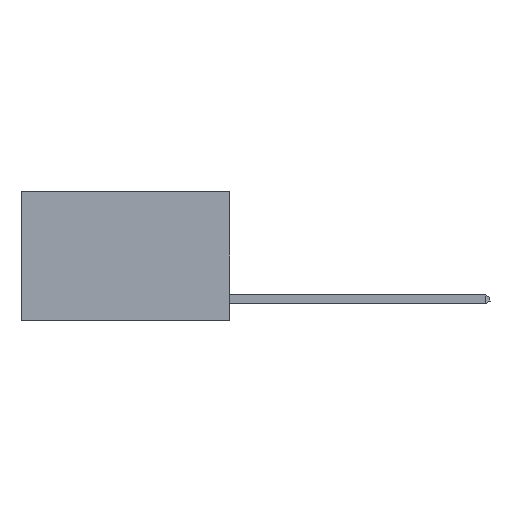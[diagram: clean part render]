
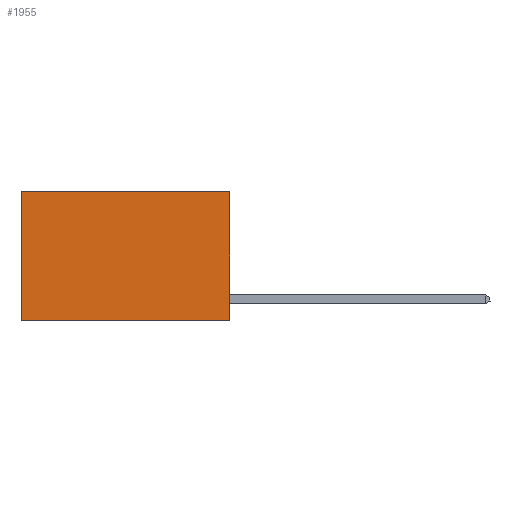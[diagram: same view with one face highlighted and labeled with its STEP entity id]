
A CAD part, left-side view. The second image highlights one B-rep face of the part: STEP entity #1955.
In plain terms, the highlighted planar face has unit normal (-1, 0, 0).
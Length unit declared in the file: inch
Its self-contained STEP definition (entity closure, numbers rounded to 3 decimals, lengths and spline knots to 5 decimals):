
#59 = LINE ( 'NONE', #3723, #6686 ) ;
#368 = DIRECTION ( 'NONE',  ( 0., 0., -1. ) ) ;
#416 = CARTESIAN_POINT ( 'NONE',  ( 0.2625, 0.6, 0. ) ) ;
#532 = VERTEX_POINT ( 'NONE', #5235 ) ;
#1898 = FACE_OUTER_BOUND ( 'NONE', #8113, .T. ) ;
#1925 = VECTOR ( 'NONE', #6934, 39.37008 ) ;
#1955 = ADVANCED_FACE ( 'NONE', ( #1898 ), #10443, .F. ) ;
#1997 = VECTOR ( 'NONE', #5068, 39.37008 ) ;
#2147 = CARTESIAN_POINT ( 'NONE',  ( 0.2625, 0., 0. ) ) ;
#2485 = AXIS2_PLACEMENT_3D ( 'NONE', #2147, #2920, #368 ) ;
#2717 = LINE ( 'NONE', #2907, #1925 ) ;
#2907 = CARTESIAN_POINT ( 'NONE',  ( 0.2625, 0., -0.37 ) ) ;
#2920 = DIRECTION ( 'NONE',  ( 1., 0., 0. ) ) ;
#3299 = ORIENTED_EDGE ( 'NONE', *, *, #6671, .F. ) ;
#3723 = CARTESIAN_POINT ( 'NONE',  ( 0.2625, 0.6, 0. ) ) ;
#4108 = ORIENTED_EDGE ( 'NONE', *, *, #7429, .T. ) ;
#4578 = VERTEX_POINT ( 'NONE', #9314 ) ;
#4613 = LINE ( 'NONE', #8494, #6379 ) ;
#5068 = DIRECTION ( 'NONE',  ( 0., 0., -1. ) ) ;
#5235 = CARTESIAN_POINT ( 'NONE',  ( 0.2625, 0.6, -0.37 ) ) ;
#6025 = DIRECTION ( 'NONE',  ( 0., 1., 0. ) ) ;
#6379 = VECTOR ( 'NONE', #6025, 39.37008 ) ;
#6627 = ORIENTED_EDGE ( 'NONE', *, *, #7870, .T. ) ;
#6668 = LINE ( 'NONE', #7596, #1997 ) ;
#6671 = EDGE_CURVE ( 'NONE', #8196, #532, #2717, .T. ) ;
#6686 = VECTOR ( 'NONE', #7843, 39.37008 ) ;
#6934 = DIRECTION ( 'NONE',  ( 0., 1., 0. ) ) ;
#7429 = EDGE_CURVE ( 'NONE', #9465, #532, #59, .T. ) ;
#7596 = CARTESIAN_POINT ( 'NONE',  ( 0.2625, 0., 0. ) ) ;
#7843 = DIRECTION ( 'NONE',  ( 0., 0., -1. ) ) ;
#7870 = EDGE_CURVE ( 'NONE', #4578, #9465, #4613, .T. ) ;
#7888 = EDGE_CURVE ( 'NONE', #4578, #8196, #6668, .T. ) ;
#8113 = EDGE_LOOP ( 'NONE', ( #4108, #3299, #10310, #6627 ) ) ;
#8174 = CARTESIAN_POINT ( 'NONE',  ( 0.2625, 0., -0.37 ) ) ;
#8196 = VERTEX_POINT ( 'NONE', #8174 ) ;
#8494 = CARTESIAN_POINT ( 'NONE',  ( 0.2625, 0., 0. ) ) ;
#9314 = CARTESIAN_POINT ( 'NONE',  ( 0.2625, 0., 0. ) ) ;
#9465 = VERTEX_POINT ( 'NONE', #416 ) ;
#10310 = ORIENTED_EDGE ( 'NONE', *, *, #7888, .F. ) ;
#10443 = PLANE ( 'NONE',  #2485 ) ;
